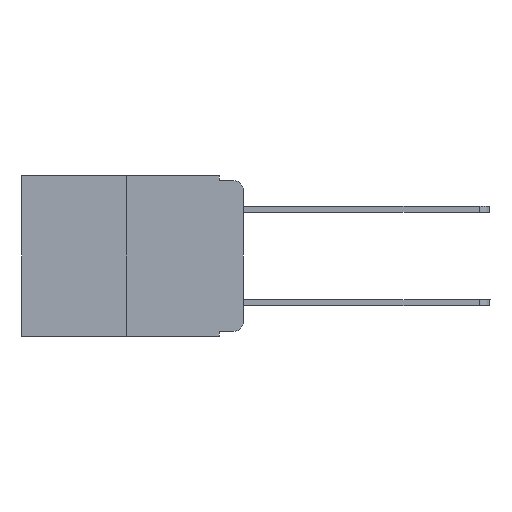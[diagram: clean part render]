
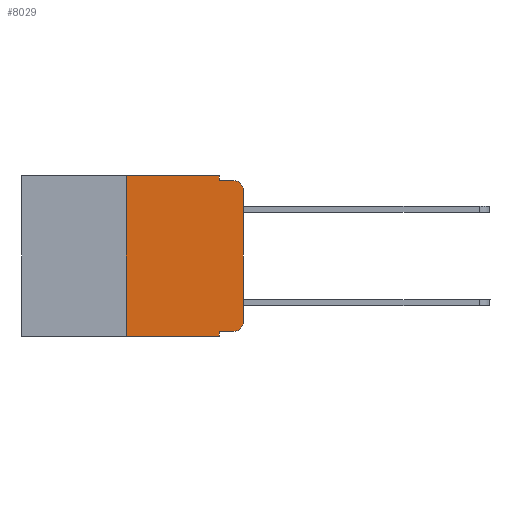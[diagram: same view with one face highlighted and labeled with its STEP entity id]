
A CAD part, left-side view. The second image highlights one B-rep face of the part: STEP entity #8029.
In plain terms, the highlighted planar face has unit normal (-1, 0, 0).
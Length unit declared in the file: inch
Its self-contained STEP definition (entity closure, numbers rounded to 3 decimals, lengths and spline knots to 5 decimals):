
#52 = VERTEX_POINT ( 'NONE', #9651 ) ;
#170 = LINE ( 'NONE', #8619, #7164 ) ;
#493 = ORIENTED_EDGE ( 'NONE', *, *, #1729, .T. ) ;
#513 = DIRECTION ( 'NONE',  ( 0., 0., -1. ) ) ;
#669 = CARTESIAN_POINT ( 'NONE',  ( 0., 0.25, 0. ) ) ;
#693 = DIRECTION ( 'NONE',  ( -1., 0., 0. ) ) ;
#1435 = CARTESIAN_POINT ( 'NONE',  ( 0., 0.051, 0. ) ) ;
#1514 = CARTESIAN_POINT ( 'NONE',  ( 0., 0.02, -0.03 ) ) ;
#1729 = EDGE_CURVE ( 'NONE', #7551, #4710, #7529, .T. ) ;
#1909 = CARTESIAN_POINT ( 'NONE',  ( 0., 0.051, -0.343 ) ) ;
#1936 = CARTESIAN_POINT ( 'NONE',  ( 0., 0.051, -0.333 ) ) ;
#2532 = LINE ( 'NONE', #9160, #12423 ) ;
#2658 = DIRECTION ( 'NONE',  ( 0., 0., -1. ) ) ;
#2672 = CARTESIAN_POINT ( 'NONE',  ( 0., 0.051, 0. ) ) ;
#2712 = CARTESIAN_POINT ( 'NONE',  ( 0., 0.02, -0.333 ) ) ;
#2722 = EDGE_CURVE ( 'NONE', #4710, #7002, #3924, .T. ) ;
#3163 = CARTESIAN_POINT ( 'NONE',  ( 0., 0.25, -0.343 ) ) ;
#3204 = CARTESIAN_POINT ( 'NONE',  ( 0., 0.02, -0.01 ) ) ;
#3269 = CARTESIAN_POINT ( 'NONE',  ( 0., 0.473, -0.343 ) ) ;
#3924 = CIRCLE ( 'NONE', #4193, 0.02 ) ;
#3928 = ORIENTED_EDGE ( 'NONE', *, *, #4014, .F. ) ;
#3952 = DIRECTION ( 'NONE',  ( 0., 0., 1. ) ) ;
#4014 = EDGE_CURVE ( 'NONE', #5502, #8395, #2532, .T. ) ;
#4045 = CARTESIAN_POINT ( 'NONE',  ( 0., 0., 0. ) ) ;
#4193 = AXIS2_PLACEMENT_3D ( 'NONE', #8574, #693, #8613 ) ;
#4437 = PLANE ( 'NONE',  #6222 ) ;
#4614 = ORIENTED_EDGE ( 'NONE', *, *, #5274, .F. ) ;
#4634 = DIRECTION ( 'NONE',  ( 0., -1., 0. ) ) ;
#4666 = DIRECTION ( 'NONE',  ( 0., 0., 1. ) ) ;
#4710 = VERTEX_POINT ( 'NONE', #2712 ) ;
#4953 = ORIENTED_EDGE ( 'NONE', *, *, #2722, .T. ) ;
#5075 = ORIENTED_EDGE ( 'NONE', *, *, #11700, .F. ) ;
#5274 = EDGE_CURVE ( 'NONE', #6603, #5502, #10992, .T. ) ;
#5387 = VERTEX_POINT ( 'NONE', #3204 ) ;
#5415 = CARTESIAN_POINT ( 'NONE',  ( 0., 0.051, -0.01 ) ) ;
#5502 = VERTEX_POINT ( 'NONE', #7354 ) ;
#5541 = DIRECTION ( 'NONE',  ( 0., 0., -1. ) ) ;
#5992 = VECTOR ( 'NONE', #10076, 39.37008 ) ;
#6078 = CARTESIAN_POINT ( 'NONE',  ( 0., 0., -0.313 ) ) ;
#6222 = AXIS2_PLACEMENT_3D ( 'NONE', #12413, #11471, #5541 ) ;
#6328 = VECTOR ( 'NONE', #10178, 39.37008 ) ;
#6361 = VECTOR ( 'NONE', #4634, 39.37008 ) ;
#6603 = VERTEX_POINT ( 'NONE', #3163 ) ;
#6792 = EDGE_CURVE ( 'NONE', #52, #5387, #10954, .T. ) ;
#6843 = ORIENTED_EDGE ( 'NONE', *, *, #9968, .T. ) ;
#7002 = VERTEX_POINT ( 'NONE', #6078 ) ;
#7105 = EDGE_CURVE ( 'NONE', #6603, #9329, #8950, .T. ) ;
#7164 = VECTOR ( 'NONE', #2658, 39.37008 ) ;
#7354 = CARTESIAN_POINT ( 'NONE',  ( 0., 0.25, 0. ) ) ;
#7377 = DIRECTION ( 'NONE',  ( 0., 0., -1. ) ) ;
#7529 = LINE ( 'NONE', #11027, #5992 ) ;
#7551 = VERTEX_POINT ( 'NONE', #1936 ) ;
#7815 = VECTOR ( 'NONE', #7377, 39.37008 ) ;
#8029 = ADVANCED_FACE ( 'NONE', ( #12504 ), #4437, .F. ) ;
#8043 = AXIS2_PLACEMENT_3D ( 'NONE', #1514, #10505, #513 ) ;
#8115 = ORIENTED_EDGE ( 'NONE', *, *, #6792, .T. ) ;
#8184 = DIRECTION ( 'NONE',  ( 0., -1., 0. ) ) ;
#8226 = LINE ( 'NONE', #8481, #6361 ) ;
#8388 = VECTOR ( 'NONE', #4666, 39.37008 ) ;
#8395 = VERTEX_POINT ( 'NONE', #2672 ) ;
#8457 = LINE ( 'NONE', #4045, #12760 ) ;
#8481 = CARTESIAN_POINT ( 'NONE',  ( 0., 0.051, -0.01 ) ) ;
#8574 = CARTESIAN_POINT ( 'NONE',  ( 0., 0.02, -0.313 ) ) ;
#8613 = DIRECTION ( 'NONE',  ( 0., 0., -1. ) ) ;
#8619 = CARTESIAN_POINT ( 'NONE',  ( 0., 0.051, 0. ) ) ;
#8950 = LINE ( 'NONE', #3269, #6328 ) ;
#9160 = CARTESIAN_POINT ( 'NONE',  ( 0., 0.473, 0. ) ) ;
#9329 = VERTEX_POINT ( 'NONE', #1909 ) ;
#9638 = LINE ( 'NONE', #1435, #7815 ) ;
#9651 = CARTESIAN_POINT ( 'NONE',  ( 0., 0., -0.03 ) ) ;
#9968 = EDGE_CURVE ( 'NONE', #7002, #52, #8457, .T. ) ;
#10076 = DIRECTION ( 'NONE',  ( 0., -1., 0. ) ) ;
#10178 = DIRECTION ( 'NONE',  ( 0., -1., 0. ) ) ;
#10234 = VERTEX_POINT ( 'NONE', #5415 ) ;
#10505 = DIRECTION ( 'NONE',  ( -1., 0., 0. ) ) ;
#10824 = EDGE_CURVE ( 'NONE', #8395, #10234, #9638, .T. ) ;
#10954 = CIRCLE ( 'NONE', #8043, 0.02 ) ;
#10992 = LINE ( 'NONE', #669, #8388 ) ;
#11027 = CARTESIAN_POINT ( 'NONE',  ( 0., 0.051, -0.333 ) ) ;
#11276 = ORIENTED_EDGE ( 'NONE', *, *, #7105, .T. ) ;
#11471 = DIRECTION ( 'NONE',  ( 1., 0., 0. ) ) ;
#11700 = EDGE_CURVE ( 'NONE', #7551, #9329, #170, .T. ) ;
#11785 = EDGE_LOOP ( 'NONE', ( #6843, #8115, #12308, #12551, #3928, #4614, #11276, #5075, #493, #4953 ) ) ;
#12308 = ORIENTED_EDGE ( 'NONE', *, *, #12355, .F. ) ;
#12355 = EDGE_CURVE ( 'NONE', #10234, #5387, #8226, .T. ) ;
#12413 = CARTESIAN_POINT ( 'NONE',  ( 0., 0.473, 0. ) ) ;
#12423 = VECTOR ( 'NONE', #8184, 39.37008 ) ;
#12504 = FACE_OUTER_BOUND ( 'NONE', #11785, .T. ) ;
#12551 = ORIENTED_EDGE ( 'NONE', *, *, #10824, .F. ) ;
#12760 = VECTOR ( 'NONE', #3952, 39.37008 ) ;
